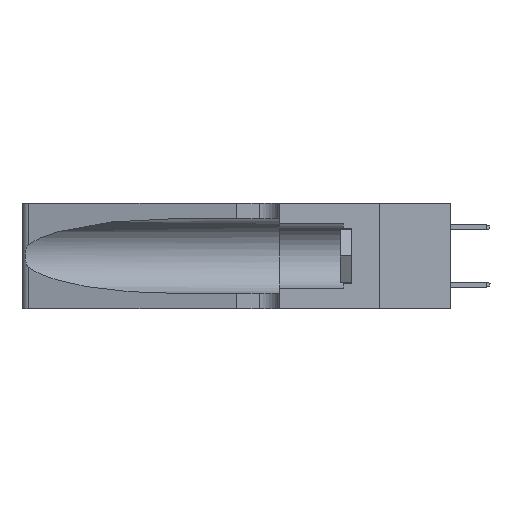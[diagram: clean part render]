
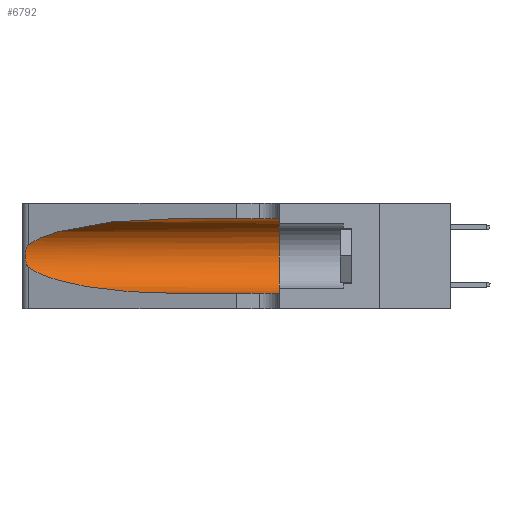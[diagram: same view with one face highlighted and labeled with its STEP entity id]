
A CAD part, left-side view. The second image highlights one B-rep face of the part: STEP entity #6792.
In plain terms, the highlighted cylindrical face has radius 3.308 mm (diameter 6.617 mm), a partial arc.
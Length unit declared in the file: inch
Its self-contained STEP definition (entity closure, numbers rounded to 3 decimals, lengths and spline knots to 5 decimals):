
#197 = EDGE_CURVE ( 'NONE', #7271, #2849, #12642, .T. ) ;
#1871 = CARTESIAN_POINT ( 'NONE',  ( 0.25487, 1.22718, 0.14631 ) ) ;
#2344 = CARTESIAN_POINT ( 'NONE',  ( 0.1305, 1.61858, 0.31525 ) ) ;
#2568 = DIRECTION ( 'NONE',  ( 0., -1., 0. ) ) ;
#2810 = EDGE_CURVE ( 'NONE', #20844, #2849, #7182, .T. ) ;
#2849 = VERTEX_POINT ( 'NONE', #4984 ) ;
#3198 = FACE_OUTER_BOUND ( 'NONE', #34445, .T. ) ;
#3699 = DIRECTION ( 'NONE',  ( 0., 0., 1. ) ) ;
#4984 = CARTESIAN_POINT ( 'NONE',  ( 0.1305, 0.35, 0.05475 ) ) ;
#5130 = DIRECTION ( 'NONE',  ( 0., -1., 0. ) ) ;
#5369 = CARTESIAN_POINT ( 'NONE',  ( 0.26075, 1.23896, 0.19203 ) ) ;
#5658 = CARTESIAN_POINT ( 'NONE',  ( 0.18966, 0.96281, 0.31525 ) ) ;
#6248 = AXIS2_PLACEMENT_3D ( 'NONE', #38395, #2568, #42249 ) ;
#6792 = ADVANCED_FACE ( 'NONE', ( #3198 ), #16284, .F. ) ;
#7182 = LINE ( 'NONE', #17454, #20264 ) ;
#7271 = VERTEX_POINT ( 'NONE', #13619 ) ;
#8820 = CARTESIAN_POINT ( 'NONE',  ( 0.25639, 1.23186, 0.15144 ) ) ;
#8885 = CARTESIAN_POINT ( 'NONE',  ( 0.25487, 1.22718, 0.22369 ) ) ;
#9479 = CARTESIAN_POINT ( 'NONE',  ( 0.25555, 1.22993, 0.14849 ) ) ;
#9493 = VERTEX_POINT ( 'NONE', #20626 ) ;
#11362 = EDGE_CURVE ( 'NONE', #20043, #7271, #25070, .T. ) ;
#11639 = CARTESIAN_POINT ( 'NONE',  ( 0.25555, 1.22994, 0.2215 ) ) ;
#12617 = ORIENTED_EDGE ( 'NONE', *, *, #11362, .F. ) ;
#12642 = CIRCLE ( 'NONE', #40675, 0.13025 ) ;
#13619 = CARTESIAN_POINT ( 'NONE',  ( 0.1305, 0.35, 0.31525 ) ) ;
#14456 = DIRECTION ( 'NONE',  ( 0., -1., 0. ) ) ;
#15270 = CARTESIAN_POINT ( 'NONE',  ( 0.25854, 1.2359, 0.20912 ) ) ;
#15330 = CARTESIAN_POINT ( 'NONE',  ( 0.2373, 1.15595, 0.28018 ) ) ;
#15483 = CARTESIAN_POINT ( 'NONE',  ( 0.25487, 1.22718, 0.14631 ) ) ;
#16284 = CYLINDRICAL_SURFACE ( 'NONE', #6248, 0.13025 ) ;
#16454 = EDGE_CURVE ( 'NONE', #20043, #9493, #19354, .T. ) ;
#17065 = ORIENTED_EDGE ( 'NONE', *, *, #16454, .T. ) ;
#17454 = CARTESIAN_POINT ( 'NONE',  ( 0.1305, 1.61858, 0.05475 ) ) ;
#18688 = CARTESIAN_POINT ( 'NONE',  ( 0.26075, 1.23896, 0.178 ) ) ;
#19354 =( BOUNDED_CURVE ( )  B_SPLINE_CURVE ( 3, ( #41058, #5658, #15330, #8885 ),
 .UNSPECIFIED., .F., .T. ) 
 B_SPLINE_CURVE_WITH_KNOTS ( ( 4, 4 ),
 ( 1.5708, 2.84003 ),
 .UNSPECIFIED. ) 
 CURVE ( )  GEOMETRIC_REPRESENTATION_ITEM ( )  RATIONAL_B_SPLINE_CURVE ( ( 1., 0.87, 0.87, 1. ) ) 
 REPRESENTATION_ITEM ( '' )  );
#19366 = CARTESIAN_POINT ( 'NONE',  ( 0.1305, 0.72297, 0.31525 ) ) ;
#19406 = ORIENTED_EDGE ( 'NONE', *, *, #19618, .T. ) ;
#19618 = EDGE_CURVE ( 'NONE', #30952, #20844, #32501, .T. ) ;
#20043 = VERTEX_POINT ( 'NONE', #19366 ) ;
#20264 = VECTOR ( 'NONE', #14456, 39.37008 ) ;
#20625 = CARTESIAN_POINT ( 'NONE',  ( 0.25487, 1.22718, 0.22369 ) ) ;
#20626 = CARTESIAN_POINT ( 'NONE',  ( 0.25487, 1.22718, 0.22369 ) ) ;
#20844 = VERTEX_POINT ( 'NONE', #40736 ) ;
#21620 = CARTESIAN_POINT ( 'NONE',  ( 0.2373, 1.15595, 0.08982 ) ) ;
#22853 = CARTESIAN_POINT ( 'NONE',  ( 0.18966, 0.96281, 0.05475 ) ) ;
#23665 = DIRECTION ( 'NONE',  ( 0., 1., 0. ) ) ;
#25070 = LINE ( 'NONE', #2344, #27449 ) ;
#25550 = CARTESIAN_POINT ( 'NONE',  ( 0.25856, 1.23593, 0.16098 ) ) ;
#27449 = VECTOR ( 'NONE', #5130, 39.37008 ) ;
#28069 = ORIENTED_EDGE ( 'NONE', *, *, #35947, .T. ) ;
#28548 = CARTESIAN_POINT ( 'NONE',  ( 0.26017, 1.23833, 0.17102 ) ) ;
#29757 = ORIENTED_EDGE ( 'NONE', *, *, #2810, .T. ) ;
#30073 = B_SPLINE_CURVE_WITH_KNOTS ( 'NONE', 3,
 ( #20625, #11639, #31987, #38208, #15270, #35420, #5369, #18688, #28548, #25550, #41845, #8820, #9479, #15483 ),
 .UNSPECIFIED., .F., .F.,
 ( 4, 2, 2, 2, 2, 2, 4 ),
 ( 0., 0.00027, 0.00053, 0.00107, 0.0016, 0.00187, 0.00214 ),
 .UNSPECIFIED. ) ;
#30952 = VERTEX_POINT ( 'NONE', #41963 ) ;
#31145 = ORIENTED_EDGE ( 'NONE', *, *, #197, .F. ) ;
#31987 = CARTESIAN_POINT ( 'NONE',  ( 0.25639, 1.23184, 0.21858 ) ) ;
#32501 =( BOUNDED_CURVE ( )  B_SPLINE_CURVE ( 3, ( #1871, #21620, #22853, #34694 ),
 .UNSPECIFIED., .F., .T. ) 
 B_SPLINE_CURVE_WITH_KNOTS ( ( 4, 4 ),
 ( 3.44316, 4.71239 ),
 .UNSPECIFIED. ) 
 CURVE ( )  GEOMETRIC_REPRESENTATION_ITEM ( )  RATIONAL_B_SPLINE_CURVE ( ( 1., 0.87, 0.87, 1. ) ) 
 REPRESENTATION_ITEM ( '' )  );
#34445 = EDGE_LOOP ( 'NONE', ( #17065, #28069, #19406, #29757, #31145, #12617 ) ) ;
#34694 = CARTESIAN_POINT ( 'NONE',  ( 0.1305, 0.72297, 0.05475 ) ) ;
#35420 = CARTESIAN_POINT ( 'NONE',  ( 0.26018, 1.23835, 0.19895 ) ) ;
#35947 = EDGE_CURVE ( 'NONE', #9493, #30952, #30073, .T. ) ;
#38208 = CARTESIAN_POINT ( 'NONE',  ( 0.25787, 1.23484, 0.2124 ) ) ;
#38395 = CARTESIAN_POINT ( 'NONE',  ( 0.1305, 1.61858, 0.185 ) ) ;
#39975 = CARTESIAN_POINT ( 'NONE',  ( 0.1305, 0.35, 0.185 ) ) ;
#40675 = AXIS2_PLACEMENT_3D ( 'NONE', #39975, #23665, #3699 ) ;
#40736 = CARTESIAN_POINT ( 'NONE',  ( 0.1305, 0.72297, 0.05475 ) ) ;
#41058 = CARTESIAN_POINT ( 'NONE',  ( 0.1305, 0.72297, 0.31525 ) ) ;
#41845 = CARTESIAN_POINT ( 'NONE',  ( 0.25789, 1.23486, 0.15765 ) ) ;
#41963 = CARTESIAN_POINT ( 'NONE',  ( 0.25487, 1.22718, 0.14631 ) ) ;
#42249 = DIRECTION ( 'NONE',  ( 0., 0., -1. ) ) ;
